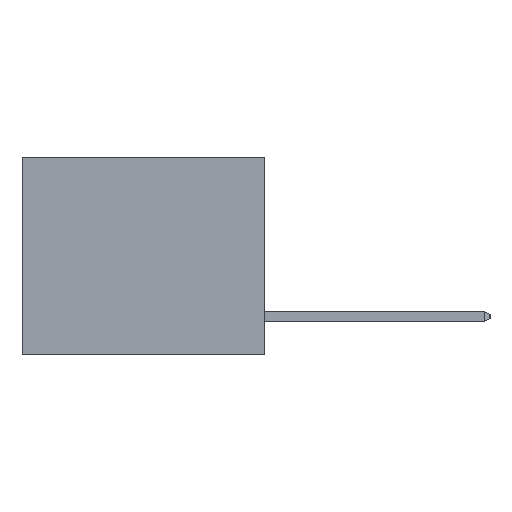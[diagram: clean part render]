
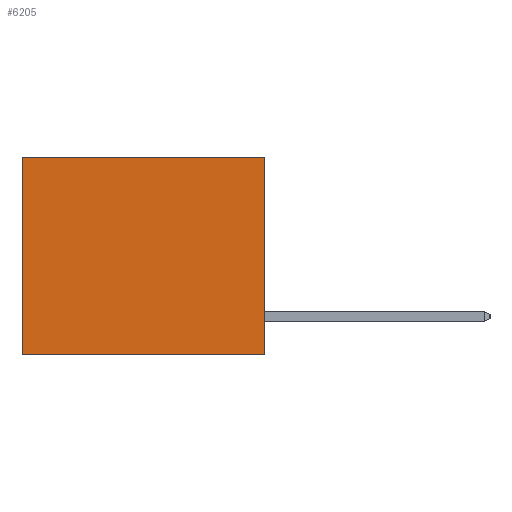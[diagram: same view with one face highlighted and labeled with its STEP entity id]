
A CAD part, left-side view. The second image highlights one B-rep face of the part: STEP entity #6205.
In plain terms, the highlighted planar face has unit normal (-1, 0, 0).
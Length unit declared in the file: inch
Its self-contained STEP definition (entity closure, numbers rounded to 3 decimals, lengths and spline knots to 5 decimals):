
#237 = LINE ( 'NONE', #3980, #8963 ) ;
#395 = DIRECTION ( 'NONE',  ( 0., 0., -1. ) ) ;
#604 = EDGE_CURVE ( 'NONE', #2751, #1279, #4202, .T. ) ;
#663 = VECTOR ( 'NONE', #8491, 39.37008 ) ;
#665 = CARTESIAN_POINT ( 'NONE',  ( 0.3165, 0., -0.49 ) ) ;
#1004 = VERTEX_POINT ( 'NONE', #7456 ) ;
#1120 = CARTESIAN_POINT ( 'NONE',  ( 0.3165, 0., 0. ) ) ;
#1279 = VERTEX_POINT ( 'NONE', #2762 ) ;
#1442 = VERTEX_POINT ( 'NONE', #8976 ) ;
#1760 = VECTOR ( 'NONE', #7035, 39.37008 ) ;
#2308 = EDGE_CURVE ( 'NONE', #1442, #1004, #8204, .T. ) ;
#2751 = VERTEX_POINT ( 'NONE', #3369 ) ;
#2762 = CARTESIAN_POINT ( 'NONE',  ( 0.3165, 0.6, 0. ) ) ;
#3310 = CARTESIAN_POINT ( 'NONE',  ( 0.3165, 0., -0.49 ) ) ;
#3369 = CARTESIAN_POINT ( 'NONE',  ( 0.3165, 0., 0. ) ) ;
#3566 = ORIENTED_EDGE ( 'NONE', *, *, #6836, .F. ) ;
#3980 = CARTESIAN_POINT ( 'NONE',  ( 0.3165, 0.6, -0.49 ) ) ;
#4202 = LINE ( 'NONE', #1120, #663 ) ;
#4209 = EDGE_CURVE ( 'NONE', #1279, #1004, #237, .T. ) ;
#5355 = ORIENTED_EDGE ( 'NONE', *, *, #604, .T. ) ;
#5580 = VECTOR ( 'NONE', #7916, 39.37008 ) ;
#5854 = EDGE_LOOP ( 'NONE', ( #8035, #8470, #3566, #5355 ) ) ;
#6205 = ADVANCED_FACE ( 'NONE', ( #6255 ), #7911, .F. ) ;
#6255 = FACE_OUTER_BOUND ( 'NONE', #5854, .T. ) ;
#6470 = DIRECTION ( 'NONE',  ( 0., 0., -1. ) ) ;
#6836 = EDGE_CURVE ( 'NONE', #2751, #1442, #7768, .T. ) ;
#7035 = DIRECTION ( 'NONE',  ( 0., 1., 0. ) ) ;
#7255 = CARTESIAN_POINT ( 'NONE',  ( 0.3165, 0., -0.49 ) ) ;
#7456 = CARTESIAN_POINT ( 'NONE',  ( 0.3165, 0.6, -0.49 ) ) ;
#7592 = AXIS2_PLACEMENT_3D ( 'NONE', #7255, #8647, #6470 ) ;
#7768 = LINE ( 'NONE', #665, #5580 ) ;
#7911 = PLANE ( 'NONE',  #7592 ) ;
#7916 = DIRECTION ( 'NONE',  ( 0., 0., -1. ) ) ;
#8035 = ORIENTED_EDGE ( 'NONE', *, *, #4209, .T. ) ;
#8204 = LINE ( 'NONE', #3310, #1760 ) ;
#8470 = ORIENTED_EDGE ( 'NONE', *, *, #2308, .F. ) ;
#8491 = DIRECTION ( 'NONE',  ( 0., 1., 0. ) ) ;
#8647 = DIRECTION ( 'NONE',  ( 1., 0., 0. ) ) ;
#8963 = VECTOR ( 'NONE', #395, 39.37008 ) ;
#8976 = CARTESIAN_POINT ( 'NONE',  ( 0.3165, 0., -0.49 ) ) ;
